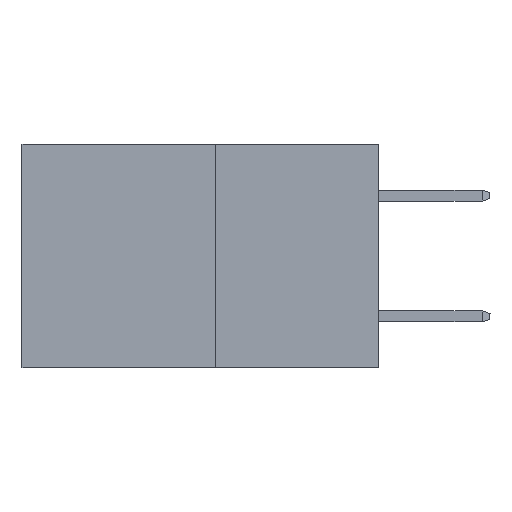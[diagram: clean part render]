
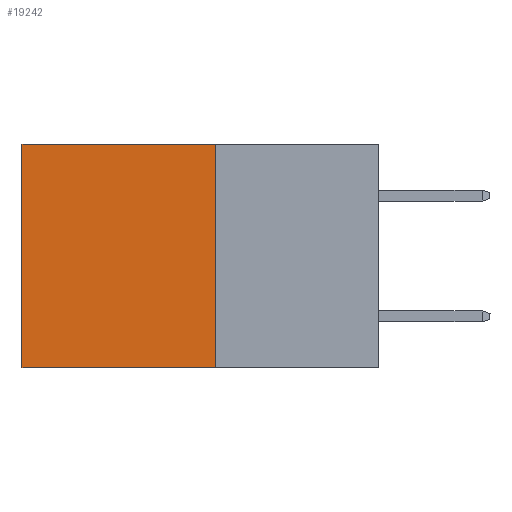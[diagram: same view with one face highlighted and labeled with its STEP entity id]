
A CAD part, left-side view. The second image highlights one B-rep face of the part: STEP entity #19242.
In plain terms, the highlighted planar face has unit normal (-1, 0, 0).
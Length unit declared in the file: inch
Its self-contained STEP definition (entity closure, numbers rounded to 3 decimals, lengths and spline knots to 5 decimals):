
#25 = CARTESIAN_POINT ( 'NONE',  ( 0.277, 0.27, -0.37 ) ) ;
#408 = EDGE_LOOP ( 'NONE', ( #11773, #7967, #14123, #13271 ) ) ;
#912 = DIRECTION ( 'NONE',  ( 1., 0., 0. ) ) ;
#1666 = LINE ( 'NONE', #25, #6213 ) ;
#2055 = DIRECTION ( 'NONE',  ( 0., 1., 0. ) ) ;
#3143 = CARTESIAN_POINT ( 'NONE',  ( 0.277, 0.27, -0.37 ) ) ;
#3670 = CARTESIAN_POINT ( 'NONE',  ( 0.277, 0.59, -0.37 ) ) ;
#4930 = EDGE_CURVE ( 'NONE', #21142, #11029, #21934, .T. ) ;
#6213 = VECTOR ( 'NONE', #2055, 39.37008 ) ;
#7967 = ORIENTED_EDGE ( 'NONE', *, *, #19684, .F. ) ;
#8014 = CARTESIAN_POINT ( 'NONE',  ( 0.277, 0.27, 0. ) ) ;
#8617 = VERTEX_POINT ( 'NONE', #3143 ) ;
#9192 = EDGE_CURVE ( 'NONE', #20484, #21142, #17065, .T. ) ;
#9235 = VECTOR ( 'NONE', #10238, 39.37008 ) ;
#9944 = CARTESIAN_POINT ( 'NONE',  ( 0.277, 0.27, 0. ) ) ;
#10044 = FACE_OUTER_BOUND ( 'NONE', #408, .T. ) ;
#10238 = DIRECTION ( 'NONE',  ( 0., 0., -1. ) ) ;
#11029 = VERTEX_POINT ( 'NONE', #3670 ) ;
#11643 = CARTESIAN_POINT ( 'NONE',  ( 0.277, 0.59, 0. ) ) ;
#11773 = ORIENTED_EDGE ( 'NONE', *, *, #4930, .T. ) ;
#12758 = DIRECTION ( 'NONE',  ( 0., 0., -1. ) ) ;
#12860 = LINE ( 'NONE', #21421, #9235 ) ;
#13006 = CARTESIAN_POINT ( 'NONE',  ( 0.277, 0.59, -0.37 ) ) ;
#13271 = ORIENTED_EDGE ( 'NONE', *, *, #9192, .T. ) ;
#14123 = ORIENTED_EDGE ( 'NONE', *, *, #15549, .F. ) ;
#14245 = DIRECTION ( 'NONE',  ( 0., 0., -1. ) ) ;
#15549 = EDGE_CURVE ( 'NONE', #20484, #8617, #12860, .T. ) ;
#16972 = VECTOR ( 'NONE', #12758, 39.37008 ) ;
#17065 = LINE ( 'NONE', #8014, #22035 ) ;
#17873 = PLANE ( 'NONE',  #20253 ) ;
#19201 = DIRECTION ( 'NONE',  ( 0., 1., 0. ) ) ;
#19242 = ADVANCED_FACE ( 'NONE', ( #10044 ), #17873, .F. ) ;
#19684 = EDGE_CURVE ( 'NONE', #8617, #11029, #1666, .T. ) ;
#20253 = AXIS2_PLACEMENT_3D ( 'NONE', #23477, #912, #14245 ) ;
#20484 = VERTEX_POINT ( 'NONE', #9944 ) ;
#21142 = VERTEX_POINT ( 'NONE', #11643 ) ;
#21421 = CARTESIAN_POINT ( 'NONE',  ( 0.277, 0.27, -0.37 ) ) ;
#21934 = LINE ( 'NONE', #13006, #16972 ) ;
#22035 = VECTOR ( 'NONE', #19201, 39.37008 ) ;
#23477 = CARTESIAN_POINT ( 'NONE',  ( 0.277, 0.27, -0.37 ) ) ;
